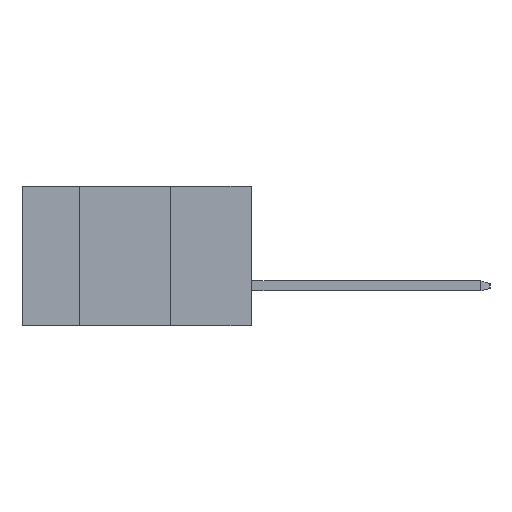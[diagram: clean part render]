
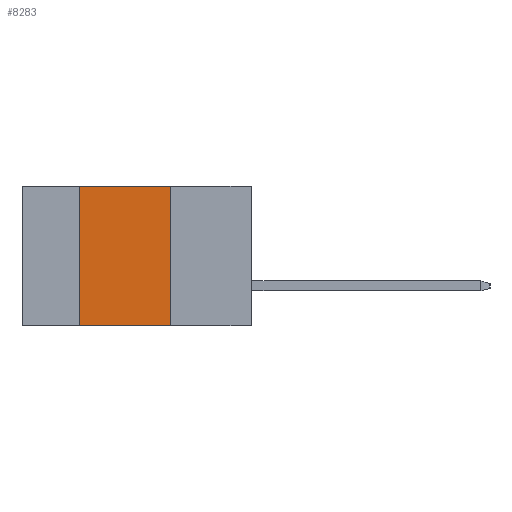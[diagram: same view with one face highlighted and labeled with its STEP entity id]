
A CAD part, left-side view. The second image highlights one B-rep face of the part: STEP entity #8283.
In plain terms, the highlighted planar face has unit normal (-1, 0, 0).
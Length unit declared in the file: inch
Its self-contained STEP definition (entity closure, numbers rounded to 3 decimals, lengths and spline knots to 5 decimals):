
#141 = FACE_OUTER_BOUND ( 'NONE', #10667, .T. ) ;
#189 = PLANE ( 'NONE',  #9043 ) ;
#1063 = VERTEX_POINT ( 'NONE', #2275 ) ;
#1700 = ORIENTED_EDGE ( 'NONE', *, *, #1836, .F. ) ;
#1779 = CARTESIAN_POINT ( 'NONE',  ( 0., 0.54, -0.437 ) ) ;
#1836 = EDGE_CURVE ( 'NONE', #9557, #3955, #8248, .T. ) ;
#1879 = LINE ( 'NONE', #2332, #2690 ) ;
#1896 = CARTESIAN_POINT ( 'NONE',  ( 0., 0.254, -0.437 ) ) ;
#2150 = CARTESIAN_POINT ( 'NONE',  ( 0., 0.72, 0. ) ) ;
#2275 = CARTESIAN_POINT ( 'NONE',  ( 0., 0.54, -0.437 ) ) ;
#2332 = CARTESIAN_POINT ( 'NONE',  ( 0., 0.72, 0. ) ) ;
#2646 = LINE ( 'NONE', #1779, #7114 ) ;
#2690 = VECTOR ( 'NONE', #4120, 39.37008 ) ;
#2724 = CARTESIAN_POINT ( 'NONE',  ( 0., 0.254, -0.437 ) ) ;
#3309 = LINE ( 'NONE', #5668, #3332 ) ;
#3332 = VECTOR ( 'NONE', #7478, 39.37008 ) ;
#3955 = VERTEX_POINT ( 'NONE', #2724 ) ;
#4120 = DIRECTION ( 'NONE',  ( 0., -1., 0. ) ) ;
#4488 = ORIENTED_EDGE ( 'NONE', *, *, #7880, .F. ) ;
#4671 = VECTOR ( 'NONE', #10807, 39.37008 ) ;
#5235 = ORIENTED_EDGE ( 'NONE', *, *, #7341, .F. ) ;
#5668 = CARTESIAN_POINT ( 'NONE',  ( 0., 0.72, -0.437 ) ) ;
#6767 = DIRECTION ( 'NONE',  ( 0., 0., -1. ) ) ;
#7114 = VECTOR ( 'NONE', #11390, 39.37008 ) ;
#7341 = EDGE_CURVE ( 'NONE', #1063, #10573, #2646, .T. ) ;
#7478 = DIRECTION ( 'NONE',  ( 0., -1., 0. ) ) ;
#7880 = EDGE_CURVE ( 'NONE', #10573, #9557, #1879, .T. ) ;
#8248 = LINE ( 'NONE', #1896, #4671 ) ;
#8283 = ADVANCED_FACE ( 'NONE', ( #141 ), #189, .F. ) ;
#8700 = ORIENTED_EDGE ( 'NONE', *, *, #9172, .T. ) ;
#9043 = AXIS2_PLACEMENT_3D ( 'NONE', #2150, #11177, #6767 ) ;
#9172 = EDGE_CURVE ( 'NONE', #1063, #3955, #3309, .T. ) ;
#9557 = VERTEX_POINT ( 'NONE', #9848 ) ;
#9673 = CARTESIAN_POINT ( 'NONE',  ( 0., 0.54, 0. ) ) ;
#9848 = CARTESIAN_POINT ( 'NONE',  ( 0., 0.254, 0. ) ) ;
#10573 = VERTEX_POINT ( 'NONE', #9673 ) ;
#10667 = EDGE_LOOP ( 'NONE', ( #1700, #4488, #5235, #8700 ) ) ;
#10807 = DIRECTION ( 'NONE',  ( 0., 0., -1. ) ) ;
#11177 = DIRECTION ( 'NONE',  ( 1., 0., 0. ) ) ;
#11390 = DIRECTION ( 'NONE',  ( 0., 0., 1. ) ) ;
